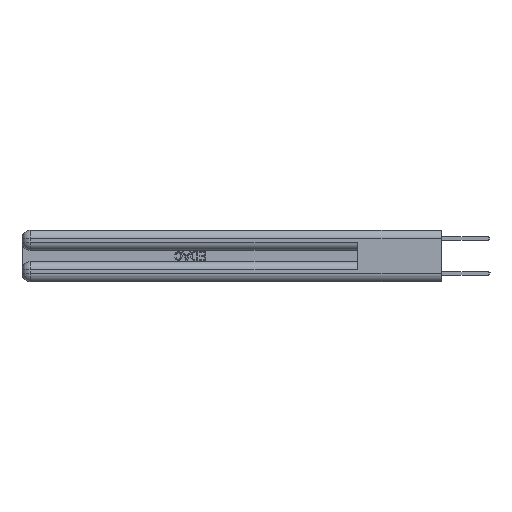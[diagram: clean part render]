
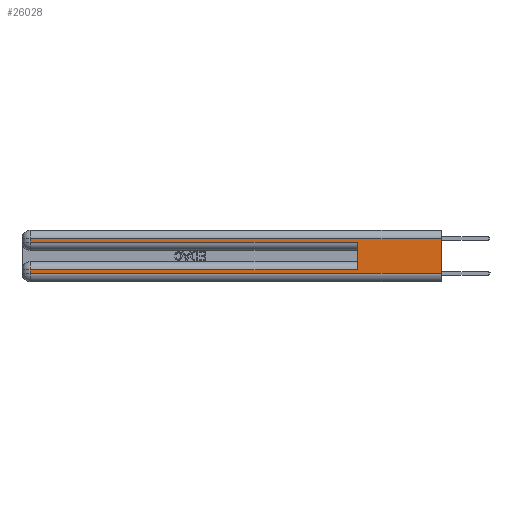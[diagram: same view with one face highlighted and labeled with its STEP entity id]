
A CAD part, left-side view. The second image highlights one B-rep face of the part: STEP entity #26028.
In plain terms, the highlighted planar face has unit normal (-1, 0, 0).
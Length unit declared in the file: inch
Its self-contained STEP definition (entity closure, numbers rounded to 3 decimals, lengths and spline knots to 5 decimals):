
#7 = CARTESIAN_POINT ( 'NONE',  ( 0., 0., 0.37 ) ) ;
#12 = LINE ( 'NONE', #12491, #14672 ) ;
#86 = CARTESIAN_POINT ( 'NONE',  ( 0., 0.6, 0.085 ) ) ;
#219 = CARTESIAN_POINT ( 'NONE',  ( 0., 2.94, 0.085 ) ) ;
#445 = CARTESIAN_POINT ( 'NONE',  ( 0., 0., 0.06 ) ) ;
#1012 = EDGE_CURVE ( 'NONE', #10219, #14790, #10757, .T. ) ;
#1874 = VECTOR ( 'NONE', #14069, 39.37008 ) ;
#2353 = LINE ( 'NONE', #16035, #19901 ) ;
#2881 = DIRECTION ( 'NONE',  ( 1., 0., 0. ) ) ;
#2902 = LINE ( 'NONE', #17393, #6208 ) ;
#3048 = LINE ( 'NONE', #7, #25568 ) ;
#3773 = AXIS2_PLACEMENT_3D ( 'NONE', #21754, #2881, #21840 ) ;
#3924 = FACE_OUTER_BOUND ( 'NONE', #14537, .T. ) ;
#4962 = VECTOR ( 'NONE', #14453, 39.37008 ) ;
#4970 = EDGE_CURVE ( 'NONE', #25075, #7471, #2902, .T. ) ;
#6076 = VERTEX_POINT ( 'NONE', #25998 ) ;
#6208 = VECTOR ( 'NONE', #6832, 39.37008 ) ;
#6832 = DIRECTION ( 'NONE',  ( 0., -1., 0. ) ) ;
#7471 = VERTEX_POINT ( 'NONE', #25081 ) ;
#7574 = LINE ( 'NONE', #17666, #4962 ) ;
#8613 = EDGE_CURVE ( 'NONE', #10219, #9216, #3048, .T. ) ;
#8779 = ORIENTED_EDGE ( 'NONE', *, *, #9349, .T. ) ;
#8973 = EDGE_CURVE ( 'NONE', #14790, #25075, #12, .T. ) ;
#9216 = VERTEX_POINT ( 'NONE', #445 ) ;
#9349 = EDGE_CURVE ( 'NONE', #25300, #6076, #2353, .T. ) ;
#10219 = VERTEX_POINT ( 'NONE', #23040 ) ;
#10757 = LINE ( 'NONE', #27443, #15787 ) ;
#11914 = ORIENTED_EDGE ( 'NONE', *, *, #8973, .T. ) ;
#12491 = CARTESIAN_POINT ( 'NONE',  ( 0., 2.94, 0.37 ) ) ;
#12511 = ORIENTED_EDGE ( 'NONE', *, *, #1012, .T. ) ;
#12861 = ORIENTED_EDGE ( 'NONE', *, *, #19028, .T. ) ;
#13641 = DIRECTION ( 'NONE',  ( 0., 0., -1. ) ) ;
#13823 = CARTESIAN_POINT ( 'NONE',  ( 0., 2.94, 0.31 ) ) ;
#14069 = DIRECTION ( 'NONE',  ( 0., 0., 1. ) ) ;
#14453 = DIRECTION ( 'NONE',  ( 0., 1., 0. ) ) ;
#14537 = EDGE_LOOP ( 'NONE', ( #21880, #12511, #11914, #18578, #17739, #18019, #8779, #12861 ) ) ;
#14672 = VECTOR ( 'NONE', #23324, 39.37008 ) ;
#14790 = VERTEX_POINT ( 'NONE', #13823 ) ;
#15787 = VECTOR ( 'NONE', #19476, 39.37008 ) ;
#15809 = EDGE_CURVE ( 'NONE', #23983, #25300, #7574, .T. ) ;
#16035 = CARTESIAN_POINT ( 'NONE',  ( 0., 2.94, 0.37 ) ) ;
#16262 = DIRECTION ( 'NONE',  ( 0., -1., 0. ) ) ;
#16896 = DIRECTION ( 'NONE',  ( 0., 0., -1. ) ) ;
#17393 = CARTESIAN_POINT ( 'NONE',  ( 0., 0., 0.285 ) ) ;
#17666 = CARTESIAN_POINT ( 'NONE',  ( 0., 0., 0.085 ) ) ;
#17739 = ORIENTED_EDGE ( 'NONE', *, *, #19112, .F. ) ;
#18019 = ORIENTED_EDGE ( 'NONE', *, *, #15809, .T. ) ;
#18445 = LINE ( 'NONE', #18638, #25737 ) ;
#18578 = ORIENTED_EDGE ( 'NONE', *, *, #4970, .T. ) ;
#18638 = CARTESIAN_POINT ( 'NONE',  ( 0., 0., 0.06 ) ) ;
#19028 = EDGE_CURVE ( 'NONE', #6076, #9216, #18445, .T. ) ;
#19112 = EDGE_CURVE ( 'NONE', #23983, #7471, #19442, .T. ) ;
#19442 = LINE ( 'NONE', #26709, #1874 ) ;
#19476 = DIRECTION ( 'NONE',  ( 0., 1., 0. ) ) ;
#19539 = PLANE ( 'NONE',  #3773 ) ;
#19901 = VECTOR ( 'NONE', #13641, 39.37008 ) ;
#21754 = CARTESIAN_POINT ( 'NONE',  ( 0., 0., 0.37 ) ) ;
#21840 = DIRECTION ( 'NONE',  ( 0., 0., -1. ) ) ;
#21880 = ORIENTED_EDGE ( 'NONE', *, *, #8613, .F. ) ;
#23040 = CARTESIAN_POINT ( 'NONE',  ( 0., 0., 0.31 ) ) ;
#23087 = CARTESIAN_POINT ( 'NONE',  ( 0., 2.94, 0.285 ) ) ;
#23324 = DIRECTION ( 'NONE',  ( 0., 0., -1. ) ) ;
#23983 = VERTEX_POINT ( 'NONE', #86 ) ;
#25075 = VERTEX_POINT ( 'NONE', #23087 ) ;
#25081 = CARTESIAN_POINT ( 'NONE',  ( 0., 0.6, 0.285 ) ) ;
#25300 = VERTEX_POINT ( 'NONE', #219 ) ;
#25568 = VECTOR ( 'NONE', #16896, 39.37008 ) ;
#25737 = VECTOR ( 'NONE', #16262, 39.37008 ) ;
#25998 = CARTESIAN_POINT ( 'NONE',  ( 0., 2.94, 0.06 ) ) ;
#26028 = ADVANCED_FACE ( 'NONE', ( #3924 ), #19539, .F. ) ;
#26709 = CARTESIAN_POINT ( 'NONE',  ( 0., 0.6, 0.145 ) ) ;
#27443 = CARTESIAN_POINT ( 'NONE',  ( 0., 0., 0.31 ) ) ;
